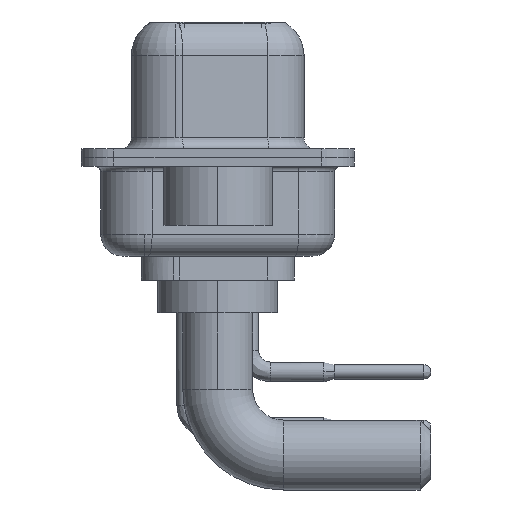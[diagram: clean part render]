
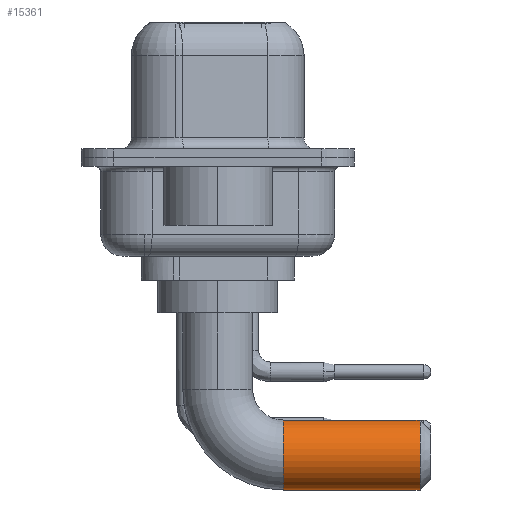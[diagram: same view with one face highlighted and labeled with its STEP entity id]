
A CAD part, left-side view. The second image highlights one B-rep face of the part: STEP entity #15361.
In plain terms, the highlighted cylindrical face has radius 1.6 mm (diameter 3.2 mm), a partial arc.
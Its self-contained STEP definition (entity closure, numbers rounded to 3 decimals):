
#126 = AXIS2_PLACEMENT_3D ( 'NONE', #10207, #18344, #8447 ) ;
#246 = DIRECTION ( 'NONE',  ( 0., -1., 0. ) ) ;
#260 = VERTEX_POINT ( 'NONE', #9819 ) ;
#452 = CARTESIAN_POINT ( 'NONE',  ( 0., -3., -6.5 ) ) ;
#598 = CARTESIAN_POINT ( 'NONE',  ( 0., -3., -4.9 ) ) ;
#1414 = LINE ( 'NONE', #4758, #17926 ) ;
#1675 = AXIS2_PLACEMENT_3D ( 'NONE', #452, #246, #12440 ) ;
#2343 = EDGE_CURVE ( 'NONE', #6519, #12321, #12874, .T. ) ;
#4616 = CARTESIAN_POINT ( 'NONE',  ( 0., -3., -8.1 ) ) ;
#4758 = CARTESIAN_POINT ( 'NONE',  ( 0., -3., -8.1 ) ) ;
#5307 = LINE ( 'NONE', #598, #7361 ) ;
#6519 = VERTEX_POINT ( 'NONE', #14119 ) ;
#7361 = VECTOR ( 'NONE', #17715, 1000. ) ;
#7549 = FACE_OUTER_BOUND ( 'NONE', #15130, .T. ) ;
#7776 = DIRECTION ( 'NONE',  ( 0., -1., 0. ) ) ;
#8447 = DIRECTION ( 'NONE',  ( 0., 0., -1. ) ) ;
#9102 = ORIENTED_EDGE ( 'NONE', *, *, #2343, .T. ) ;
#9122 = AXIS2_PLACEMENT_3D ( 'NONE', #12962, #16753, #14761 ) ;
#9819 = CARTESIAN_POINT ( 'NONE',  ( 0., -3., -4.9 ) ) ;
#10207 = CARTESIAN_POINT ( 'NONE',  ( 0., -9.25, -6.5 ) ) ;
#10835 = VERTEX_POINT ( 'NONE', #4616 ) ;
#11254 = CIRCLE ( 'NONE', #1675, 1.6 ) ;
#11787 = EDGE_CURVE ( 'NONE', #10835, #6519, #1414, .T. ) ;
#12321 = VERTEX_POINT ( 'NONE', #13499 ) ;
#12440 = DIRECTION ( 'NONE',  ( -1., 0., 0. ) ) ;
#12874 = CIRCLE ( 'NONE', #126, 1.6 ) ;
#12962 = CARTESIAN_POINT ( 'NONE',  ( 0., -3., -6.5 ) ) ;
#13499 = CARTESIAN_POINT ( 'NONE',  ( 0., -9.25, -4.9 ) ) ;
#14119 = CARTESIAN_POINT ( 'NONE',  ( 0., -9.25, -8.1 ) ) ;
#14761 = DIRECTION ( 'NONE',  ( 0., 0., -1. ) ) ;
#15130 = EDGE_LOOP ( 'NONE', ( #19914, #16107, #21561, #9102 ) ) ;
#15361 = ADVANCED_FACE ( 'NONE', ( #7549 ), #17868, .T. ) ;
#15527 = EDGE_CURVE ( 'NONE', #260, #12321, #5307, .T. ) ;
#15990 = EDGE_CURVE ( 'NONE', #260, #10835, #11254, .T. ) ;
#16107 = ORIENTED_EDGE ( 'NONE', *, *, #15990, .T. ) ;
#16753 = DIRECTION ( 'NONE',  ( 0., -1., 0. ) ) ;
#17715 = DIRECTION ( 'NONE',  ( 0., -1., 0. ) ) ;
#17868 = CYLINDRICAL_SURFACE ( 'NONE', #9122, 1.6 ) ;
#17926 = VECTOR ( 'NONE', #7776, 1000. ) ;
#18344 = DIRECTION ( 'NONE',  ( 0., 1., 0. ) ) ;
#19914 = ORIENTED_EDGE ( 'NONE', *, *, #15527, .F. ) ;
#21561 = ORIENTED_EDGE ( 'NONE', *, *, #11787, .T. ) ;
